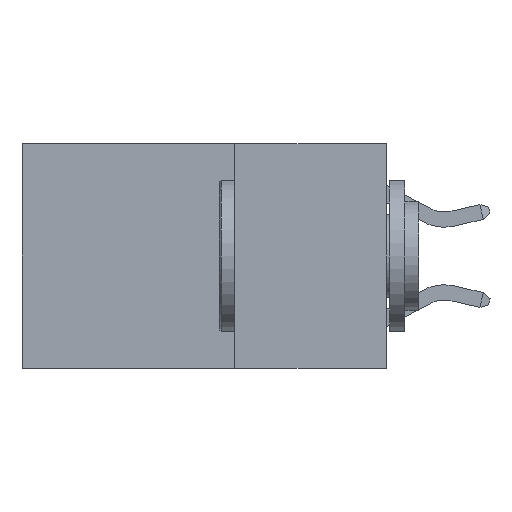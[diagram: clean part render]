
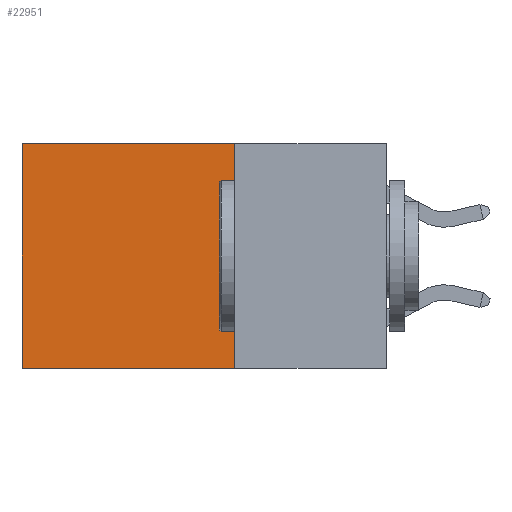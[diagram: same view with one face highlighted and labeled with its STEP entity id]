
A CAD part, left-side view. The second image highlights one B-rep face of the part: STEP entity #22951.
In plain terms, the highlighted planar face has unit normal (-1, 0, 0).
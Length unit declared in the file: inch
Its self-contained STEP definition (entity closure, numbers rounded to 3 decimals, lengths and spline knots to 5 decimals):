
#119 = EDGE_CURVE ( 'NONE', #21196, #361, #9560, .T. ) ;
#361 = VERTEX_POINT ( 'NONE', #10913 ) ;
#1561 = LINE ( 'NONE', #23211, #21092 ) ;
#2033 = VERTEX_POINT ( 'NONE', #11772 ) ;
#3600 = DIRECTION ( 'NONE',  ( 0., 0., -1. ) ) ;
#4394 = VECTOR ( 'NONE', #20043, 39.37008 ) ;
#5277 = ORIENTED_EDGE ( 'NONE', *, *, #21705, .T. ) ;
#7487 = ORIENTED_EDGE ( 'NONE', *, *, #11324, .F. ) ;
#8013 = VERTEX_POINT ( 'NONE', #14813 ) ;
#8643 = VECTOR ( 'NONE', #8902, 39.37008 ) ;
#8902 = DIRECTION ( 'NONE',  ( 0., 1., 0. ) ) ;
#9560 = LINE ( 'NONE', #14156, #4394 ) ;
#10913 = CARTESIAN_POINT ( 'NONE',  ( 0.2625, 0.6, 0. ) ) ;
#11324 = EDGE_CURVE ( 'NONE', #21196, #2033, #17614, .T. ) ;
#11328 = CARTESIAN_POINT ( 'NONE',  ( 0.2625, 0.25, 0. ) ) ;
#11566 = DIRECTION ( 'NONE',  ( 0., 0., -1. ) ) ;
#11627 = ORIENTED_EDGE ( 'NONE', *, *, #16656, .F. ) ;
#11772 = CARTESIAN_POINT ( 'NONE',  ( 0.2625, 0.25, -0.37 ) ) ;
#11825 = VECTOR ( 'NONE', #22895, 39.37008 ) ;
#14156 = CARTESIAN_POINT ( 'NONE',  ( 0.2625, 0.25, 0. ) ) ;
#14813 = CARTESIAN_POINT ( 'NONE',  ( 0.2625, 0.6, -0.37 ) ) ;
#15246 = DIRECTION ( 'NONE',  ( 1., 0., 0. ) ) ;
#16656 = EDGE_CURVE ( 'NONE', #2033, #8013, #23505, .T. ) ;
#17614 = LINE ( 'NONE', #20981, #11825 ) ;
#20043 = DIRECTION ( 'NONE',  ( 0., 1., 0. ) ) ;
#20554 = CARTESIAN_POINT ( 'NONE',  ( 0.2625, 0.25, -0.37 ) ) ;
#20981 = CARTESIAN_POINT ( 'NONE',  ( 0.2625, 0.25, 0. ) ) ;
#21055 = PLANE ( 'NONE',  #22606 ) ;
#21092 = VECTOR ( 'NONE', #11566, 39.37008 ) ;
#21147 = EDGE_LOOP ( 'NONE', ( #5277, #11627, #7487, #23365 ) ) ;
#21196 = VERTEX_POINT ( 'NONE', #22476 ) ;
#21705 = EDGE_CURVE ( 'NONE', #361, #8013, #1561, .T. ) ;
#22476 = CARTESIAN_POINT ( 'NONE',  ( 0.2625, 0.25, 0. ) ) ;
#22606 = AXIS2_PLACEMENT_3D ( 'NONE', #11328, #15246, #3600 ) ;
#22895 = DIRECTION ( 'NONE',  ( 0., 0., -1. ) ) ;
#22951 = ADVANCED_FACE ( 'NONE', ( #24639 ), #21055, .F. ) ;
#23211 = CARTESIAN_POINT ( 'NONE',  ( 0.2625, 0.6, 0. ) ) ;
#23365 = ORIENTED_EDGE ( 'NONE', *, *, #119, .T. ) ;
#23505 = LINE ( 'NONE', #20554, #8643 ) ;
#24639 = FACE_OUTER_BOUND ( 'NONE', #21147, .T. ) ;
